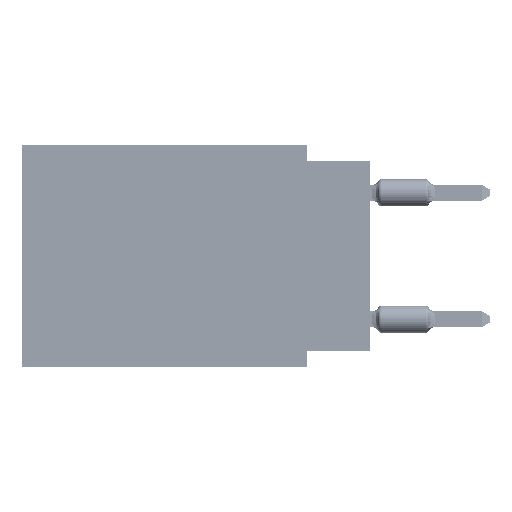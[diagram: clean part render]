
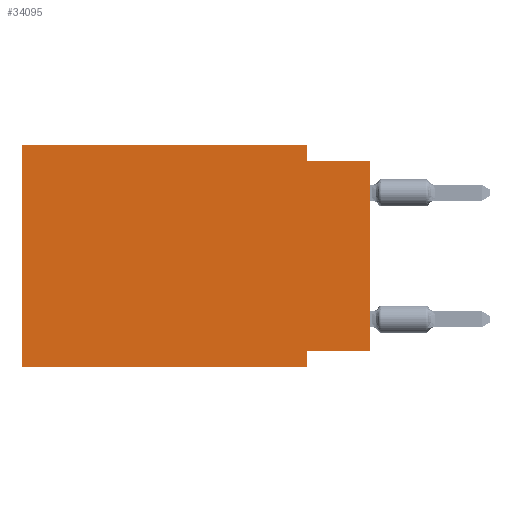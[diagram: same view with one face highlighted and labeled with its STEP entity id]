
A CAD part, left-side view. The second image highlights one B-rep face of the part: STEP entity #34095.
In plain terms, the highlighted planar face has unit normal (-1, 0, 0).
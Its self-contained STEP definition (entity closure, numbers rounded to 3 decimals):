
#907 = CARTESIAN_POINT ( 'NONE',  ( 0., 0., 0. ) ) ;
#1588 = DIRECTION ( 'NONE',  ( 0., 1., 0. ) ) ;
#3428 = LINE ( 'NONE', #19869, #37462 ) ;
#4072 = LINE ( 'NONE', #11283, #55289 ) ;
#4705 = EDGE_CURVE ( 'NONE', #42675, #23559, #73074, .T. ) ;
#5232 = ORIENTED_EDGE ( 'NONE', *, *, #68490, .F. ) ;
#5958 = LINE ( 'NONE', #32137, #27063 ) ;
#7509 = EDGE_CURVE ( 'NONE', #84136, #43323, #4072, .T. ) ;
#10130 = DIRECTION ( 'NONE',  ( 0., 0., -1. ) ) ;
#11207 = VECTOR ( 'NONE', #44508, 1000. ) ;
#11283 = CARTESIAN_POINT ( 'NONE',  ( 0., 0., -0.635 ) ) ;
#12632 = CARTESIAN_POINT ( 'NONE',  ( 0., 2.54, 0. ) ) ;
#19665 = DIRECTION ( 'NONE',  ( 0., -1., 0. ) ) ;
#19869 = CARTESIAN_POINT ( 'NONE',  ( 0., 2.54, -8.89 ) ) ;
#19896 = VERTEX_POINT ( 'NONE', #28174 ) ;
#20654 = CARTESIAN_POINT ( 'NONE',  ( 0., 13.97, -8.89 ) ) ;
#21902 = CARTESIAN_POINT ( 'NONE',  ( 0., 13.97, 0. ) ) ;
#22056 = ORIENTED_EDGE ( 'NONE', *, *, #40149, .F. ) ;
#22898 = DIRECTION ( 'NONE',  ( 0., 0., -1. ) ) ;
#23559 = VERTEX_POINT ( 'NONE', #21902 ) ;
#23911 = CARTESIAN_POINT ( 'NONE',  ( 0., 13.97, 0. ) ) ;
#24034 = CARTESIAN_POINT ( 'NONE',  ( 0., 2.54, -8.89 ) ) ;
#25398 = VECTOR ( 'NONE', #56399, 1000. ) ;
#26477 = VECTOR ( 'NONE', #96711, 1000. ) ;
#27063 = VECTOR ( 'NONE', #54736, 1000. ) ;
#28158 = ORIENTED_EDGE ( 'NONE', *, *, #60150, .T. ) ;
#28174 = CARTESIAN_POINT ( 'NONE',  ( 0., 2.54, 0. ) ) ;
#31621 = FACE_OUTER_BOUND ( 'NONE', #61360, .T. ) ;
#32054 = VERTEX_POINT ( 'NONE', #55060 ) ;
#32137 = CARTESIAN_POINT ( 'NONE',  ( 0., 13.97, 0. ) ) ;
#33816 = VECTOR ( 'NONE', #1588, 1000. ) ;
#34095 = ADVANCED_FACE ( 'NONE', ( #31621 ), #62966, .F. ) ;
#37462 = VECTOR ( 'NONE', #10130, 1000. ) ;
#40149 = EDGE_CURVE ( 'NONE', #83239, #32054, #54528, .T. ) ;
#42675 = VERTEX_POINT ( 'NONE', #81251 ) ;
#43323 = VERTEX_POINT ( 'NONE', #48141 ) ;
#43543 = ORIENTED_EDGE ( 'NONE', *, *, #52570, .T. ) ;
#44508 = DIRECTION ( 'NONE',  ( 0., 0., -1. ) ) ;
#44971 = ORIENTED_EDGE ( 'NONE', *, *, #68308, .F. ) ;
#48141 = CARTESIAN_POINT ( 'NONE',  ( 0., 0., -0.635 ) ) ;
#49831 = DIRECTION ( 'NONE',  ( 0., -1., 0. ) ) ;
#52570 = EDGE_CURVE ( 'NONE', #83239, #43323, #87058, .T. ) ;
#53735 = DIRECTION ( 'NONE',  ( 1., 0., 0. ) ) ;
#54528 = LINE ( 'NONE', #94097, #33816 ) ;
#54736 = DIRECTION ( 'NONE',  ( 0., -1., 0. ) ) ;
#55060 = CARTESIAN_POINT ( 'NONE',  ( 0., 2.54, -8.255 ) ) ;
#55289 = VECTOR ( 'NONE', #49831, 1000. ) ;
#56399 = DIRECTION ( 'NONE',  ( 0., 0., 1. ) ) ;
#57834 = VERTEX_POINT ( 'NONE', #24034 ) ;
#59639 = AXIS2_PLACEMENT_3D ( 'NONE', #23911, #53735, #22898 ) ;
#60150 = EDGE_CURVE ( 'NONE', #42675, #57834, #90050, .T. ) ;
#60726 = VECTOR ( 'NONE', #19665, 1000. ) ;
#60977 = CARTESIAN_POINT ( 'NONE',  ( 0., 0., -8.255 ) ) ;
#61360 = EDGE_LOOP ( 'NONE', ( #43543, #89369, #5232, #71190, #88129, #28158, #44971, #22056 ) ) ;
#62966 = PLANE ( 'NONE',  #59639 ) ;
#65361 = CARTESIAN_POINT ( 'NONE',  ( 0., 13.97, 0. ) ) ;
#68308 = EDGE_CURVE ( 'NONE', #32054, #57834, #3428, .T. ) ;
#68490 = EDGE_CURVE ( 'NONE', #19896, #84136, #83039, .T. ) ;
#71190 = ORIENTED_EDGE ( 'NONE', *, *, #86781, .F. ) ;
#73074 = LINE ( 'NONE', #65361, #26477 ) ;
#81251 = CARTESIAN_POINT ( 'NONE',  ( 0., 13.97, -8.89 ) ) ;
#83039 = LINE ( 'NONE', #12632, #11207 ) ;
#83239 = VERTEX_POINT ( 'NONE', #60977 ) ;
#84136 = VERTEX_POINT ( 'NONE', #90738 ) ;
#86781 = EDGE_CURVE ( 'NONE', #23559, #19896, #5958, .T. ) ;
#87058 = LINE ( 'NONE', #907, #25398 ) ;
#88129 = ORIENTED_EDGE ( 'NONE', *, *, #4705, .F. ) ;
#89369 = ORIENTED_EDGE ( 'NONE', *, *, #7509, .F. ) ;
#90050 = LINE ( 'NONE', #20654, #60726 ) ;
#90738 = CARTESIAN_POINT ( 'NONE',  ( 0., 2.54, -0.635 ) ) ;
#94097 = CARTESIAN_POINT ( 'NONE',  ( 0., 0., -8.255 ) ) ;
#96711 = DIRECTION ( 'NONE',  ( 0., 0., 1. ) ) ;
